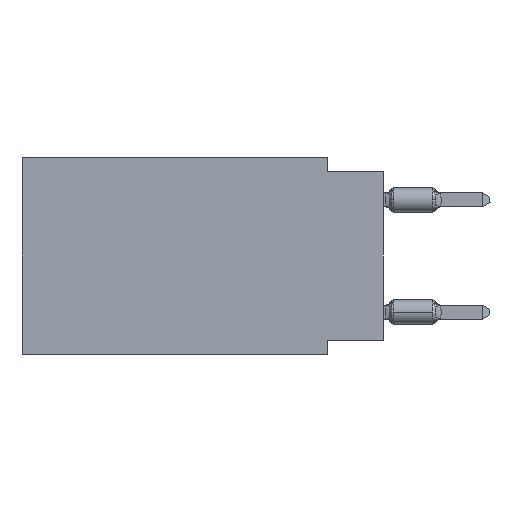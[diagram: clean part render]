
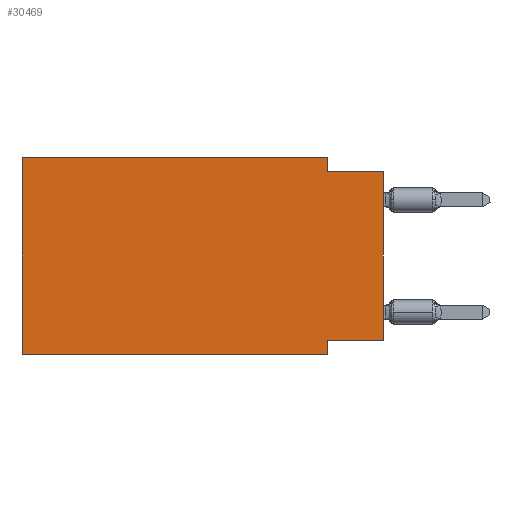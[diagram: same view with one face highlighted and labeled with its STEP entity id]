
A CAD part, left-side view. The second image highlights one B-rep face of the part: STEP entity #30469.
In plain terms, the highlighted planar face has unit normal (-1, 0, 0).
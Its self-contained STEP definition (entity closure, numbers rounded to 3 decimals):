
#405 = CARTESIAN_POINT ( 'NONE',  ( 0., 16.383, 0. ) ) ;
#1507 = ORIENTED_EDGE ( 'NONE', *, *, #44559, .F. ) ;
#3107 = VECTOR ( 'NONE', #52268, 1000. ) ;
#3175 = VERTEX_POINT ( 'NONE', #4739 ) ;
#3861 = VERTEX_POINT ( 'NONE', #12876 ) ;
#4486 = VECTOR ( 'NONE', #47068, 1000. ) ;
#4739 = CARTESIAN_POINT ( 'NONE',  ( 0., 2.54, -8.89 ) ) ;
#5389 = DIRECTION ( 'NONE',  ( 0., -1., 0. ) ) ;
#11557 = CARTESIAN_POINT ( 'NONE',  ( 0., 16.383, -8.89 ) ) ;
#12876 = CARTESIAN_POINT ( 'NONE',  ( 0., 2.54, -0.635 ) ) ;
#13092 = FACE_OUTER_BOUND ( 'NONE', #42086, .T. ) ;
#13476 = ORIENTED_EDGE ( 'NONE', *, *, #37390, .F. ) ;
#13529 = LINE ( 'NONE', #29917, #36758 ) ;
#13546 = ORIENTED_EDGE ( 'NONE', *, *, #13911, .F. ) ;
#13747 = VECTOR ( 'NONE', #45535, 1000. ) ;
#13911 = EDGE_CURVE ( 'NONE', #21719, #40187, #33742, .T. ) ;
#15633 = VECTOR ( 'NONE', #17154, 1000. ) ;
#15798 = VECTOR ( 'NONE', #48794, 1000. ) ;
#16112 = DIRECTION ( 'NONE',  ( 0., -1., 0. ) ) ;
#16464 = ORIENTED_EDGE ( 'NONE', *, *, #16661, .T. ) ;
#16661 = EDGE_CURVE ( 'NONE', #35164, #43928, #39923, .T. ) ;
#17154 = DIRECTION ( 'NONE',  ( 0., 1., 0. ) ) ;
#18355 = EDGE_CURVE ( 'NONE', #36226, #3175, #13529, .T. ) ;
#18714 = VECTOR ( 'NONE', #5389, 1000. ) ;
#20100 = ORIENTED_EDGE ( 'NONE', *, *, #18355, .F. ) ;
#21719 = VERTEX_POINT ( 'NONE', #51610 ) ;
#21922 = PLANE ( 'NONE',  #37239 ) ;
#28433 = VECTOR ( 'NONE', #16112, 1000. ) ;
#28478 = CARTESIAN_POINT ( 'NONE',  ( 0., 0., -0.635 ) ) ;
#29254 = CARTESIAN_POINT ( 'NONE',  ( 0., 0., -8.255 ) ) ;
#29464 = ORIENTED_EDGE ( 'NONE', *, *, #41918, .F. ) ;
#29717 = CARTESIAN_POINT ( 'NONE',  ( 0., 16.383, 0. ) ) ;
#29917 = CARTESIAN_POINT ( 'NONE',  ( 0., 2.54, -8.89 ) ) ;
#30259 = DIRECTION ( 'NONE',  ( 1., 0., 0. ) ) ;
#30422 = EDGE_CURVE ( 'NONE', #32724, #21719, #44496, .T. ) ;
#30469 = ADVANCED_FACE ( 'NONE', ( #13092 ), #21922, .F. ) ;
#32724 = VERTEX_POINT ( 'NONE', #46511 ) ;
#33439 = DIRECTION ( 'NONE',  ( 0., 0., -1. ) ) ;
#33742 = LINE ( 'NONE', #405, #13747 ) ;
#33757 = ORIENTED_EDGE ( 'NONE', *, *, #45120, .T. ) ;
#34903 = CARTESIAN_POINT ( 'NONE',  ( 0., 2.54, -8.255 ) ) ;
#35164 = VERTEX_POINT ( 'NONE', #37738 ) ;
#35179 = LINE ( 'NONE', #43235, #18714 ) ;
#35794 = CARTESIAN_POINT ( 'NONE',  ( 0., 2.54, 0. ) ) ;
#35930 = CARTESIAN_POINT ( 'NONE',  ( 0., 16.383, 0. ) ) ;
#36034 = CARTESIAN_POINT ( 'NONE',  ( 0., 2.54, 0. ) ) ;
#36226 = VERTEX_POINT ( 'NONE', #34903 ) ;
#36758 = VECTOR ( 'NONE', #33439, 1000. ) ;
#37239 = AXIS2_PLACEMENT_3D ( 'NONE', #29717, #30259, #46077 ) ;
#37390 = EDGE_CURVE ( 'NONE', #3861, #43928, #35179, .T. ) ;
#37738 = CARTESIAN_POINT ( 'NONE',  ( 0., 0., -8.255 ) ) ;
#39881 = ORIENTED_EDGE ( 'NONE', *, *, #30422, .F. ) ;
#39923 = LINE ( 'NONE', #48252, #3107 ) ;
#40187 = VERTEX_POINT ( 'NONE', #36034 ) ;
#41918 = EDGE_CURVE ( 'NONE', #35164, #36226, #49912, .T. ) ;
#42086 = EDGE_LOOP ( 'NONE', ( #16464, #13476, #1507, #13546, #39881, #33757, #20100, #29464 ) ) ;
#43235 = CARTESIAN_POINT ( 'NONE',  ( 0., 0., -0.635 ) ) ;
#43928 = VERTEX_POINT ( 'NONE', #28478 ) ;
#44496 = LINE ( 'NONE', #35930, #15798 ) ;
#44559 = EDGE_CURVE ( 'NONE', #40187, #3861, #51899, .T. ) ;
#44567 = LINE ( 'NONE', #11557, #28433 ) ;
#45120 = EDGE_CURVE ( 'NONE', #32724, #3175, #44567, .T. ) ;
#45535 = DIRECTION ( 'NONE',  ( 0., -1., 0. ) ) ;
#46077 = DIRECTION ( 'NONE',  ( 0., 0., -1. ) ) ;
#46511 = CARTESIAN_POINT ( 'NONE',  ( 0., 16.383, -8.89 ) ) ;
#47068 = DIRECTION ( 'NONE',  ( 0., 0., -1. ) ) ;
#48252 = CARTESIAN_POINT ( 'NONE',  ( 0., 0., 0. ) ) ;
#48794 = DIRECTION ( 'NONE',  ( 0., 0., 1. ) ) ;
#49912 = LINE ( 'NONE', #29254, #15633 ) ;
#51610 = CARTESIAN_POINT ( 'NONE',  ( 0., 16.383, 0. ) ) ;
#51899 = LINE ( 'NONE', #35794, #4486 ) ;
#52268 = DIRECTION ( 'NONE',  ( 0., 0., 1. ) ) ;
